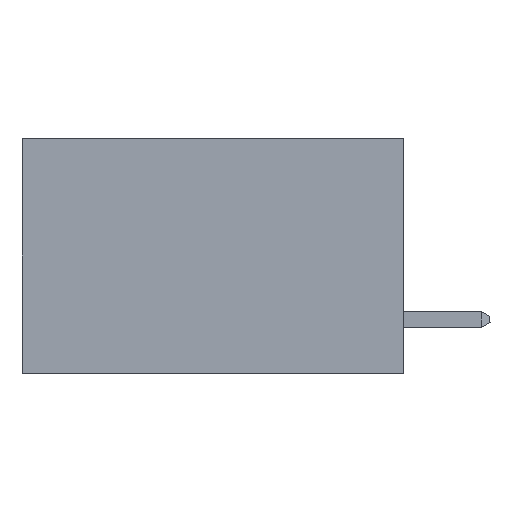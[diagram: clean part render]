
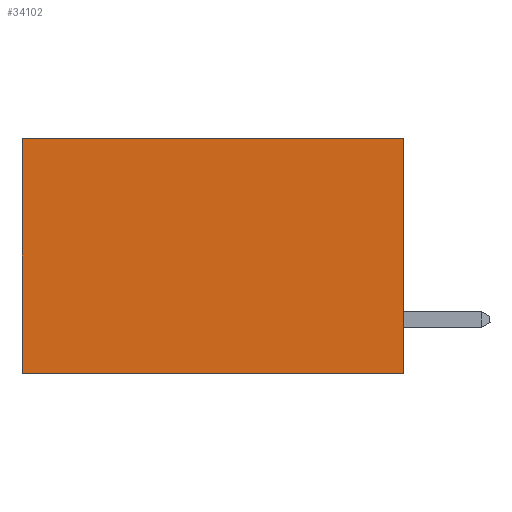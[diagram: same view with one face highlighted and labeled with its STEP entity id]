
A CAD part, left-side view. The second image highlights one B-rep face of the part: STEP entity #34102.
In plain terms, the highlighted planar face has unit normal (-1, 0, 0).
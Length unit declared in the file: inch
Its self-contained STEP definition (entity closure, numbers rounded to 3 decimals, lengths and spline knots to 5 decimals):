
#532 = VECTOR ( 'NONE', #17966, 39.37008 ) ;
#677 = LINE ( 'NONE', #17239, #17499 ) ;
#1011 = CARTESIAN_POINT ( 'NONE',  ( 0.2875, 0., 0. ) ) ;
#1551 = LINE ( 'NONE', #13148, #12723 ) ;
#1711 = VECTOR ( 'NONE', #13678, 39.37008 ) ;
#2676 = DIRECTION ( 'NONE',  ( 0., 1., 0. ) ) ;
#4035 = VERTEX_POINT ( 'NONE', #8608 ) ;
#5389 = CARTESIAN_POINT ( 'NONE',  ( 0.2875, 0.6, 0. ) ) ;
#6310 = ORIENTED_EDGE ( 'NONE', *, *, #12309, .F. ) ;
#7547 = CARTESIAN_POINT ( 'NONE',  ( 0.2875, 0., -0.37 ) ) ;
#8066 = VERTEX_POINT ( 'NONE', #27142 ) ;
#8608 = CARTESIAN_POINT ( 'NONE',  ( 0.2875, 0., 0. ) ) ;
#9003 = LINE ( 'NONE', #5389, #1711 ) ;
#9873 = VERTEX_POINT ( 'NONE', #32414 ) ;
#10852 = AXIS2_PLACEMENT_3D ( 'NONE', #1011, #33622, #25623 ) ;
#11685 = ORIENTED_EDGE ( 'NONE', *, *, #29906, .T. ) ;
#12309 = EDGE_CURVE ( 'NONE', #9873, #26989, #18230, .T. ) ;
#12723 = VECTOR ( 'NONE', #2676, 39.37008 ) ;
#13148 = CARTESIAN_POINT ( 'NONE',  ( 0.2875, 0., 0. ) ) ;
#13678 = DIRECTION ( 'NONE',  ( 0., 0., -1. ) ) ;
#14871 = PLANE ( 'NONE',  #10852 ) ;
#16657 = FACE_OUTER_BOUND ( 'NONE', #25813, .T. ) ;
#16882 = DIRECTION ( 'NONE',  ( 0., 0., -1. ) ) ;
#17220 = EDGE_CURVE ( 'NONE', #4035, #8066, #1551, .T. ) ;
#17239 = CARTESIAN_POINT ( 'NONE',  ( 0.2875, 0., 0. ) ) ;
#17499 = VECTOR ( 'NONE', #16882, 39.37008 ) ;
#17966 = DIRECTION ( 'NONE',  ( 0., 1., 0. ) ) ;
#18230 = LINE ( 'NONE', #7547, #532 ) ;
#19514 = ORIENTED_EDGE ( 'NONE', *, *, #17220, .T. ) ;
#25531 = EDGE_CURVE ( 'NONE', #4035, #9873, #677, .T. ) ;
#25623 = DIRECTION ( 'NONE',  ( 0., 0., -1. ) ) ;
#25813 = EDGE_LOOP ( 'NONE', ( #11685, #6310, #32799, #19514 ) ) ;
#26989 = VERTEX_POINT ( 'NONE', #35120 ) ;
#27142 = CARTESIAN_POINT ( 'NONE',  ( 0.2875, 0.6, 0. ) ) ;
#29906 = EDGE_CURVE ( 'NONE', #8066, #26989, #9003, .T. ) ;
#32414 = CARTESIAN_POINT ( 'NONE',  ( 0.2875, 0., -0.37 ) ) ;
#32799 = ORIENTED_EDGE ( 'NONE', *, *, #25531, .F. ) ;
#33622 = DIRECTION ( 'NONE',  ( 1., 0., 0. ) ) ;
#34102 = ADVANCED_FACE ( 'NONE', ( #16657 ), #14871, .F. ) ;
#35120 = CARTESIAN_POINT ( 'NONE',  ( 0.2875, 0.6, -0.37 ) ) ;
